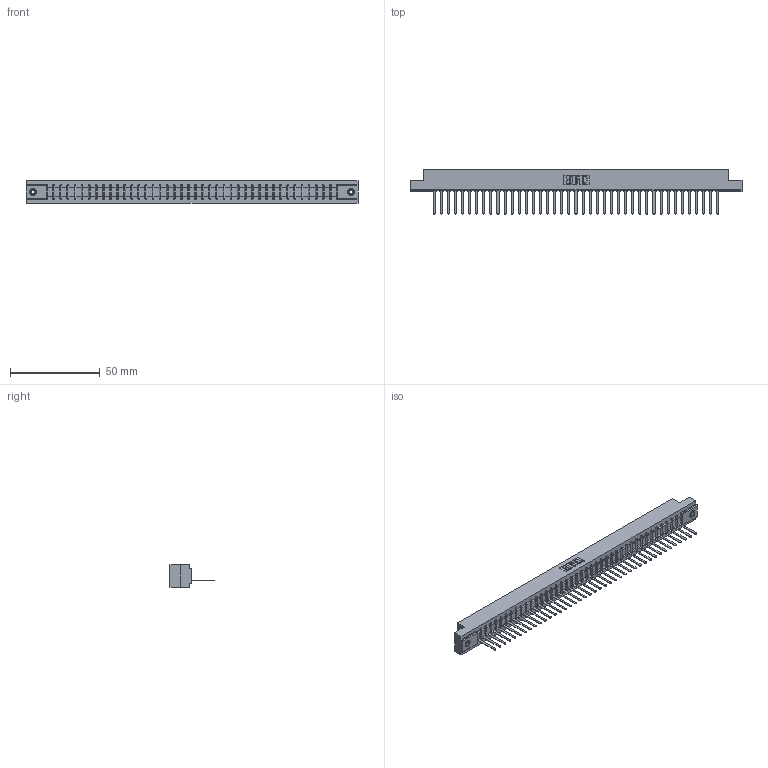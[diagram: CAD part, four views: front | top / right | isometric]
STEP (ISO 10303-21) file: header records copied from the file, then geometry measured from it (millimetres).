
FILE_DESCRIPTION (( 'STEP AP203' ), '1' );
FILE_NAME ('307-041-441-108.STEP', '2020-09-29T15:58:38', ( '' ), ( '' ), 'SwSTEP 2.0', 'SolidWorks 2020', '' );
FILE_SCHEMA (( 'CONFIG_CONTROL_DESIGN' ));
Length unit declared in the file: inch
Products named in the file (4): 307-290-002_541; 307-041-441-108; 307 Part_.156 Dia Mounting Holes; 345-250-001_345-250-003-102
Assembly tree (44 placements, depth 2):
  307-041-441-108
    307 Part_.156 Dia Mounting Holes
    307-290-002_541  x41
    345-250-001_345-250-003-102  x2
Bounding box: 185.47 x 24.59 x 12.7 mm (x, y, z)
Volume: 19949.5 mm3; surface area: 25825.9 mm2
Topology: 44 solids, 44 shells, 3254 faces, 9971 edges, 6526 vertices
Faces by surface type: plane 1947, cylinder 1207, sphere 84, cone 12, torus 4
Entity records: 37175 total; most frequent: CARTESIAN_POINT 6251, ORIENTED_EDGE 6234, DIRECTION 6083, EDGE_CURVE 3117, VECTOR 2387, LINE 2387, VERTEX_POINT 2016, AXIS2_PLACEMENT_3D 1848
